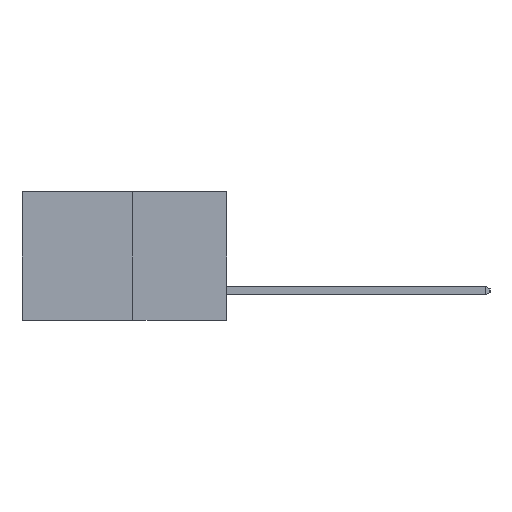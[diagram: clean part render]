
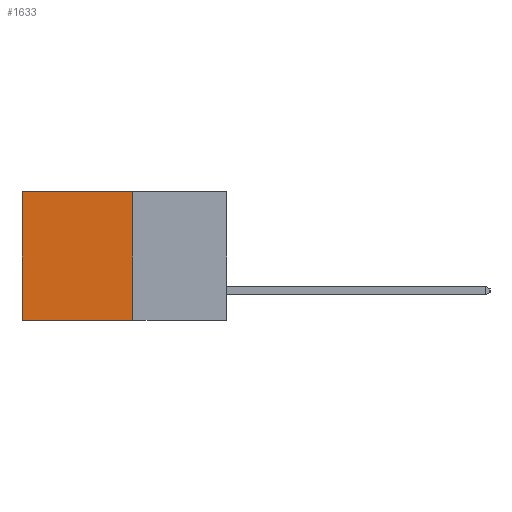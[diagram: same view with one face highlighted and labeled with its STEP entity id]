
A CAD part, left-side view. The second image highlights one B-rep face of the part: STEP entity #1633.
In plain terms, the highlighted planar face has unit normal (-1, 0, 0).
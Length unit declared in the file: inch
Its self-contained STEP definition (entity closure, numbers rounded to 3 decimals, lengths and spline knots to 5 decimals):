
#36 = ORIENTED_EDGE ( 'NONE', *, *, #15204, .T. ) ;
#381 = CARTESIAN_POINT ( 'NONE',  ( 0.277, 0.27, -0.37 ) ) ;
#1051 = LINE ( 'NONE', #13675, #13191 ) ;
#1303 = CARTESIAN_POINT ( 'NONE',  ( 0.277, 0.59, -0.37 ) ) ;
#1633 = ADVANCED_FACE ( 'NONE', ( #8216 ), #5878, .F. ) ;
#1935 = DIRECTION ( 'NONE',  ( 0., 1., 0. ) ) ;
#1967 = CARTESIAN_POINT ( 'NONE',  ( 0.277, 0.27, 0. ) ) ;
#2266 = DIRECTION ( 'NONE',  ( 0., 1., 0. ) ) ;
#2687 = VECTOR ( 'NONE', #1935, 39.37008 ) ;
#3762 = VERTEX_POINT ( 'NONE', #15739 ) ;
#4720 = DIRECTION ( 'NONE',  ( 0., 0., -1. ) ) ;
#4837 = EDGE_LOOP ( 'NONE', ( #36, #7551, #5022, #14930 ) ) ;
#5022 = ORIENTED_EDGE ( 'NONE', *, *, #11108, .F. ) ;
#5408 = EDGE_CURVE ( 'NONE', #10251, #3762, #15872, .T. ) ;
#5596 = DIRECTION ( 'NONE',  ( 0., 0., -1. ) ) ;
#5598 = DIRECTION ( 'NONE',  ( 1., 0., 0. ) ) ;
#5641 = CARTESIAN_POINT ( 'NONE',  ( 0.277, 0.27, -0.37 ) ) ;
#5878 = PLANE ( 'NONE',  #13469 ) ;
#6792 = CARTESIAN_POINT ( 'NONE',  ( 0.277, 0.27, 0. ) ) ;
#6969 = VERTEX_POINT ( 'NONE', #1303 ) ;
#7147 = VERTEX_POINT ( 'NONE', #381 ) ;
#7551 = ORIENTED_EDGE ( 'NONE', *, *, #9293, .F. ) ;
#8216 = FACE_OUTER_BOUND ( 'NONE', #4837, .T. ) ;
#9285 = LINE ( 'NONE', #15861, #12174 ) ;
#9291 = LINE ( 'NONE', #9788, #12583 ) ;
#9293 = EDGE_CURVE ( 'NONE', #7147, #6969, #9291, .T. ) ;
#9788 = CARTESIAN_POINT ( 'NONE',  ( 0.277, 0.27, -0.37 ) ) ;
#10028 = DIRECTION ( 'NONE',  ( 0., 0., -1. ) ) ;
#10251 = VERTEX_POINT ( 'NONE', #6792 ) ;
#11108 = EDGE_CURVE ( 'NONE', #10251, #7147, #9285, .T. ) ;
#12174 = VECTOR ( 'NONE', #4720, 39.37008 ) ;
#12583 = VECTOR ( 'NONE', #2266, 39.37008 ) ;
#13191 = VECTOR ( 'NONE', #10028, 39.37008 ) ;
#13469 = AXIS2_PLACEMENT_3D ( 'NONE', #5641, #5598, #5596 ) ;
#13675 = CARTESIAN_POINT ( 'NONE',  ( 0.277, 0.59, -0.37 ) ) ;
#14930 = ORIENTED_EDGE ( 'NONE', *, *, #5408, .T. ) ;
#15204 = EDGE_CURVE ( 'NONE', #3762, #6969, #1051, .T. ) ;
#15739 = CARTESIAN_POINT ( 'NONE',  ( 0.277, 0.59, 0. ) ) ;
#15861 = CARTESIAN_POINT ( 'NONE',  ( 0.277, 0.27, -0.37 ) ) ;
#15872 = LINE ( 'NONE', #1967, #2687 ) ;
